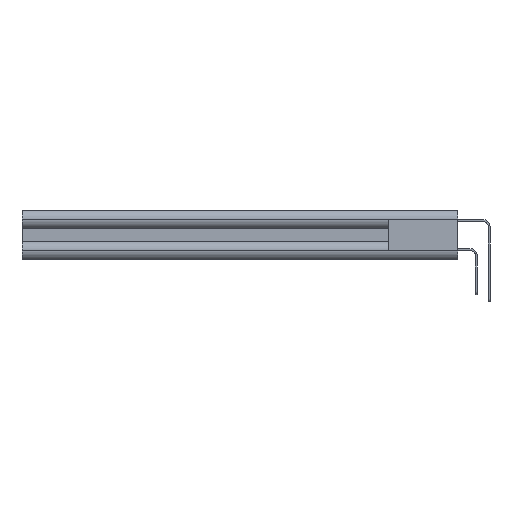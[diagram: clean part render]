
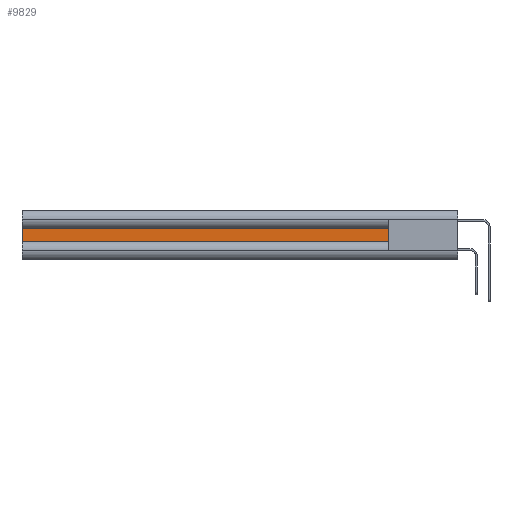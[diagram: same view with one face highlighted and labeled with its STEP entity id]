
A CAD part, left-side view. The second image highlights one B-rep face of the part: STEP entity #9829.
In plain terms, the highlighted planar face has unit normal (-1, 0, 0).
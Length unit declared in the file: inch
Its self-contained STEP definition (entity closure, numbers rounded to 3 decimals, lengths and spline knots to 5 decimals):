
#42 = VECTOR ( 'NONE', #20396, 39.37008 ) ;
#173 = VERTEX_POINT ( 'NONE', #13888 ) ;
#333 = DIRECTION ( 'NONE',  ( 1., 0., 0. ) ) ;
#605 = LINE ( 'NONE', #9469, #42 ) ;
#742 = LINE ( 'NONE', #5339, #10491 ) ;
#1377 = CARTESIAN_POINT ( 'NONE',  ( 0.044, 0.37012, -0.0465 ) ) ;
#1797 = CARTESIAN_POINT ( 'NONE',  ( 0.044, 3., -0.0465 ) ) ;
#1853 = EDGE_LOOP ( 'NONE', ( #2214, #19442, #12627, #16093 ) ) ;
#2214 = ORIENTED_EDGE ( 'NONE', *, *, #13242, .T. ) ;
#3234 = DIRECTION ( 'NONE',  ( 0., 1., 0. ) ) ;
#3636 = VERTEX_POINT ( 'NONE', #7823 ) ;
#3652 = DIRECTION ( 'NONE',  ( 0., 0., -1. ) ) ;
#5339 = CARTESIAN_POINT ( 'NONE',  ( 0.044, 0.473, -0.0465 ) ) ;
#5372 = VERTEX_POINT ( 'NONE', #9631 ) ;
#7823 = CARTESIAN_POINT ( 'NONE',  ( 0.044, 0.473, -0.0465 ) ) ;
#7873 = LINE ( 'NONE', #1797, #12161 ) ;
#9469 = CARTESIAN_POINT ( 'NONE',  ( 0.044, 0.37012, 0.0465 ) ) ;
#9483 = CARTESIAN_POINT ( 'NONE',  ( 0.044, 0.37012, -0.0465 ) ) ;
#9631 = CARTESIAN_POINT ( 'NONE',  ( 0.044, 3., -0.0465 ) ) ;
#9829 = ADVANCED_FACE ( 'NONE', ( #17643 ), #22256, .F. ) ;
#10491 = VECTOR ( 'NONE', #18101, 39.37008 ) ;
#12161 = VECTOR ( 'NONE', #3652, 39.37008 ) ;
#12208 = VERTEX_POINT ( 'NONE', #21927 ) ;
#12627 = ORIENTED_EDGE ( 'NONE', *, *, #12951, .F. ) ;
#12951 = EDGE_CURVE ( 'NONE', #3636, #5372, #20947, .T. ) ;
#13139 = DIRECTION ( 'NONE',  ( 0., 0., -1. ) ) ;
#13242 = EDGE_CURVE ( 'NONE', #12208, #173, #605, .T. ) ;
#13888 = CARTESIAN_POINT ( 'NONE',  ( 0.044, 3., 0.0465 ) ) ;
#16093 = ORIENTED_EDGE ( 'NONE', *, *, #16475, .F. ) ;
#16475 = EDGE_CURVE ( 'NONE', #12208, #3636, #742, .T. ) ;
#17213 = AXIS2_PLACEMENT_3D ( 'NONE', #9483, #333, #13139 ) ;
#17643 = FACE_OUTER_BOUND ( 'NONE', #1853, .T. ) ;
#18101 = DIRECTION ( 'NONE',  ( 0., 0., -1. ) ) ;
#19442 = ORIENTED_EDGE ( 'NONE', *, *, #20666, .T. ) ;
#20367 = VECTOR ( 'NONE', #3234, 39.37008 ) ;
#20396 = DIRECTION ( 'NONE',  ( 0., 1., 0. ) ) ;
#20666 = EDGE_CURVE ( 'NONE', #173, #5372, #7873, .T. ) ;
#20947 = LINE ( 'NONE', #1377, #20367 ) ;
#21927 = CARTESIAN_POINT ( 'NONE',  ( 0.044, 0.473, 0.0465 ) ) ;
#22256 = PLANE ( 'NONE',  #17213 ) ;
